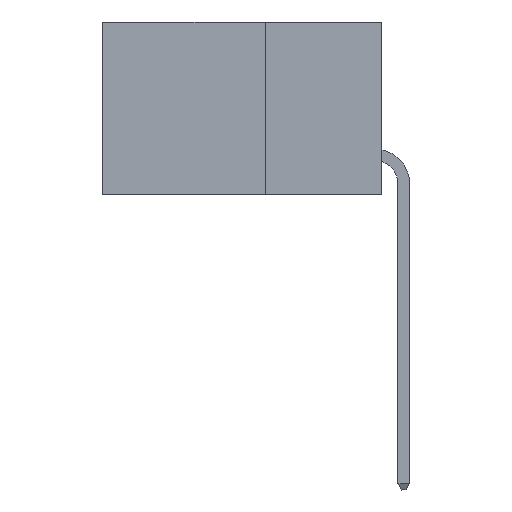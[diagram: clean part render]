
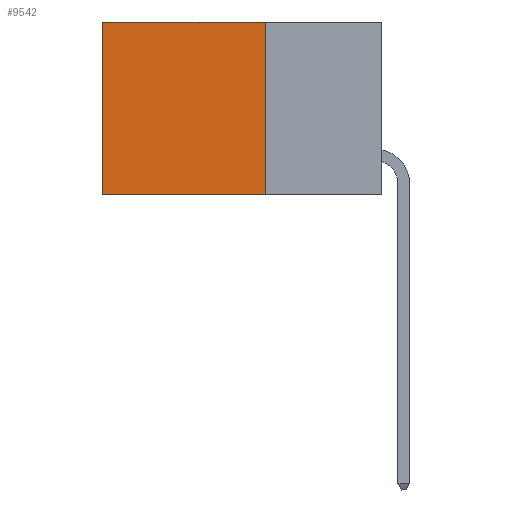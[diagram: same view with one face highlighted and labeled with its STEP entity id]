
A CAD part, left-side view. The second image highlights one B-rep face of the part: STEP entity #9542.
In plain terms, the highlighted planar face has unit normal (-1, 0, 0).
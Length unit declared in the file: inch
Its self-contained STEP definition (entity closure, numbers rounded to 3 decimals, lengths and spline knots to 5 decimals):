
#1483 = CARTESIAN_POINT ( 'NONE',  ( 0.2875, 0.6, 0. ) ) ;
#1988 = ORIENTED_EDGE ( 'NONE', *, *, #10494, .T. ) ;
#2078 = CARTESIAN_POINT ( 'NONE',  ( 0.2875, 0.25, -0.37 ) ) ;
#2368 = CARTESIAN_POINT ( 'NONE',  ( 0.2875, 0.25, 0. ) ) ;
#2454 = ORIENTED_EDGE ( 'NONE', *, *, #16711, .F. ) ;
#2650 = VERTEX_POINT ( 'NONE', #2368 ) ;
#2911 = VECTOR ( 'NONE', #10760, 39.37008 ) ;
#2945 = VECTOR ( 'NONE', #18180, 39.37008 ) ;
#2969 = DIRECTION ( 'NONE',  ( 0., 0., -1. ) ) ;
#3355 = LINE ( 'NONE', #9364, #2911 ) ;
#3936 = CARTESIAN_POINT ( 'NONE',  ( 0.2875, 0.25, 0. ) ) ;
#4974 = LINE ( 'NONE', #7699, #12183 ) ;
#5193 = CARTESIAN_POINT ( 'NONE',  ( 0.2875, 0.25, 0. ) ) ;
#5780 = VERTEX_POINT ( 'NONE', #2078 ) ;
#6138 = ORIENTED_EDGE ( 'NONE', *, *, #7187, .T. ) ;
#6299 = LINE ( 'NONE', #3936, #2945 ) ;
#7187 = EDGE_CURVE ( 'NONE', #14644, #13001, #4974, .T. ) ;
#7699 = CARTESIAN_POINT ( 'NONE',  ( 0.2875, 0.6, 0. ) ) ;
#8692 = PLANE ( 'NONE',  #13990 ) ;
#9364 = CARTESIAN_POINT ( 'NONE',  ( 0.2875, 0.25, -0.37 ) ) ;
#9370 = VECTOR ( 'NONE', #15198, 39.37008 ) ;
#9542 = ADVANCED_FACE ( 'NONE', ( #10321 ), #8692, .F. ) ;
#10321 = FACE_OUTER_BOUND ( 'NONE', #11787, .T. ) ;
#10494 = EDGE_CURVE ( 'NONE', #2650, #14644, #16948, .T. ) ;
#10760 = DIRECTION ( 'NONE',  ( 0., 1., 0. ) ) ;
#11598 = DIRECTION ( 'NONE',  ( 1., 0., 0. ) ) ;
#11787 = EDGE_LOOP ( 'NONE', ( #6138, #2454, #17117, #1988 ) ) ;
#12183 = VECTOR ( 'NONE', #17675, 39.37008 ) ;
#13001 = VERTEX_POINT ( 'NONE', #15299 ) ;
#13990 = AXIS2_PLACEMENT_3D ( 'NONE', #14360, #11598, #2969 ) ;
#14343 = EDGE_CURVE ( 'NONE', #2650, #5780, #6299, .T. ) ;
#14360 = CARTESIAN_POINT ( 'NONE',  ( 0.2875, 0.25, 0. ) ) ;
#14644 = VERTEX_POINT ( 'NONE', #1483 ) ;
#15198 = DIRECTION ( 'NONE',  ( 0., 1., 0. ) ) ;
#15299 = CARTESIAN_POINT ( 'NONE',  ( 0.2875, 0.6, -0.37 ) ) ;
#16711 = EDGE_CURVE ( 'NONE', #5780, #13001, #3355, .T. ) ;
#16948 = LINE ( 'NONE', #5193, #9370 ) ;
#17117 = ORIENTED_EDGE ( 'NONE', *, *, #14343, .F. ) ;
#17675 = DIRECTION ( 'NONE',  ( 0., 0., -1. ) ) ;
#18180 = DIRECTION ( 'NONE',  ( 0., 0., -1. ) ) ;
